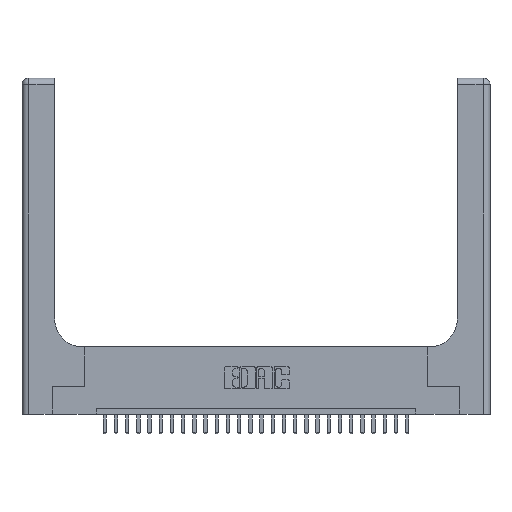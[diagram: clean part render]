
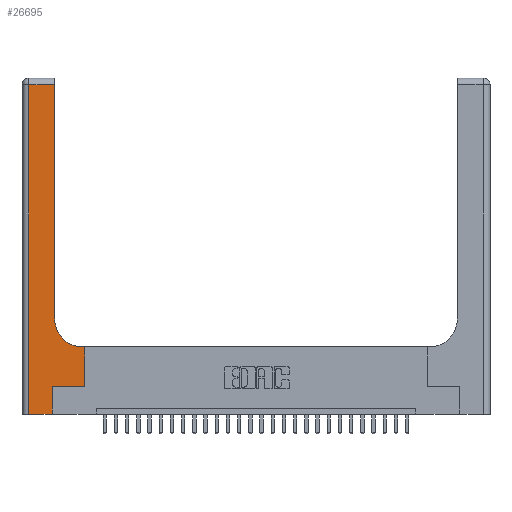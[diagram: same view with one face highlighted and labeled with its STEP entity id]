
A CAD part, top view. The second image highlights one B-rep face of the part: STEP entity #26695.
In plain terms, the highlighted planar face has unit normal (0, 0, 1).
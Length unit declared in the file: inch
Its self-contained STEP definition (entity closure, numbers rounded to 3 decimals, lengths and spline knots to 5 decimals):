
#1019 = ORIENTED_EDGE ( 'NONE', *, *, #23453, .T. ) ;
#1664 = ORIENTED_EDGE ( 'NONE', *, *, #26947, .T. ) ;
#1747 = DIRECTION ( 'NONE',  ( 1., 0., 0. ) ) ;
#2376 = LINE ( 'NONE', #21621, #3713 ) ;
#3713 = VECTOR ( 'NONE', #15261, 39.37008 ) ;
#3734 = CARTESIAN_POINT ( 'NONE',  ( 0.269, 0.25, 0.37 ) ) ;
#3906 = EDGE_CURVE ( 'NONE', #19540, #4794, #2376, .T. ) ;
#4467 = VECTOR ( 'NONE', #18921, 39.37008 ) ;
#4679 = VECTOR ( 'NONE', #12614, 39.37008 ) ;
#4794 = VERTEX_POINT ( 'NONE', #17191 ) ;
#4954 = EDGE_CURVE ( 'NONE', #4794, #5631, #6091, .T. ) ;
#5137 = ORIENTED_EDGE ( 'NONE', *, *, #26342, .T. ) ;
#5205 = DIRECTION ( 'NONE',  ( 0., 1., 0. ) ) ;
#5344 = CARTESIAN_POINT ( 'NONE',  ( 0.5415, 0.6, 0.37 ) ) ;
#5631 = VERTEX_POINT ( 'NONE', #7781 ) ;
#6091 = LINE ( 'NONE', #27931, #4679 ) ;
#6381 = DIRECTION ( 'NONE',  ( -1., 0., 0. ) ) ;
#7465 = VERTEX_POINT ( 'NONE', #10535 ) ;
#7767 = AXIS2_PLACEMENT_3D ( 'NONE', #19415, #8532, #6381 ) ;
#7781 = CARTESIAN_POINT ( 'NONE',  ( 0.269, 0., 0.37 ) ) ;
#8532 = DIRECTION ( 'NONE',  ( 0., 0., -1. ) ) ;
#9071 = DIRECTION ( 'NONE',  ( 0., 0., -1. ) ) ;
#9159 = DIRECTION ( 'NONE',  ( 1., 0., 0. ) ) ;
#9258 = EDGE_CURVE ( 'NONE', #5631, #19264, #20163, .T. ) ;
#9343 = LINE ( 'NONE', #24771, #26045 ) ;
#9934 = CARTESIAN_POINT ( 'NONE',  ( 0.06, 2.94, 0.37 ) ) ;
#10535 = CARTESIAN_POINT ( 'NONE',  ( 0.5585, 0.25, 0.37 ) ) ;
#10834 = CARTESIAN_POINT ( 'NONE',  ( 0.2915, 0.85, 0.37 ) ) ;
#10840 = DIRECTION ( 'NONE',  ( -1., 0., 0. ) ) ;
#11137 = ORIENTED_EDGE ( 'NONE', *, *, #9258, .T. ) ;
#11182 = ORIENTED_EDGE ( 'NONE', *, *, #4954, .T. ) ;
#12565 = LINE ( 'NONE', #18956, #19994 ) ;
#12614 = DIRECTION ( 'NONE',  ( 1., 0., 0. ) ) ;
#12843 = CARTESIAN_POINT ( 'NONE',  ( 0., 2.94, 0.37 ) ) ;
#13458 = VECTOR ( 'NONE', #5205, 39.37008 ) ;
#13619 = CARTESIAN_POINT ( 'NONE',  ( 0.5415, 0.85, 0.37 ) ) ;
#14384 = VERTEX_POINT ( 'NONE', #5344 ) ;
#14420 = VECTOR ( 'NONE', #10840, 39.37008 ) ;
#15104 = EDGE_CURVE ( 'NONE', #19264, #7465, #17779, .T. ) ;
#15176 = PLANE ( 'NONE',  #7767 ) ;
#15261 = DIRECTION ( 'NONE',  ( 0., -1., 0. ) ) ;
#16485 = CIRCLE ( 'NONE', #18891, 0.25 ) ;
#17094 = CARTESIAN_POINT ( 'NONE',  ( 0.5585, 0.6, 0.37 ) ) ;
#17191 = CARTESIAN_POINT ( 'NONE',  ( 0.06, 0., 0.37 ) ) ;
#17556 = CARTESIAN_POINT ( 'NONE',  ( 0.269, 0.25, 0.37 ) ) ;
#17679 = ORIENTED_EDGE ( 'NONE', *, *, #3906, .T. ) ;
#17779 = LINE ( 'NONE', #3734, #21870 ) ;
#18028 = VERTEX_POINT ( 'NONE', #10834 ) ;
#18075 = ORIENTED_EDGE ( 'NONE', *, *, #27725, .T. ) ;
#18619 = EDGE_LOOP ( 'NONE', ( #1019, #18075, #17679, #11182, #11137, #25982, #1664, #5137, #21457 ) ) ;
#18891 = AXIS2_PLACEMENT_3D ( 'NONE', #13619, #9071, #9159 ) ;
#18921 = DIRECTION ( 'NONE',  ( 0., 1., 0. ) ) ;
#18956 = CARTESIAN_POINT ( 'NONE',  ( 0.2915, 3., 0.37 ) ) ;
#19226 = LINE ( 'NONE', #20341, #13458 ) ;
#19264 = VERTEX_POINT ( 'NONE', #17556 ) ;
#19415 = CARTESIAN_POINT ( 'NONE',  ( 0., 3., 0.37 ) ) ;
#19540 = VERTEX_POINT ( 'NONE', #9934 ) ;
#19994 = VECTOR ( 'NONE', #27735, 39.37008 ) ;
#20163 = LINE ( 'NONE', #27996, #4467 ) ;
#20341 = CARTESIAN_POINT ( 'NONE',  ( 0.5585, 0.25, 0.37 ) ) ;
#20575 = VERTEX_POINT ( 'NONE', #25002 ) ;
#21457 = ORIENTED_EDGE ( 'NONE', *, *, #26749, .T. ) ;
#21553 = LINE ( 'NONE', #12843, #14420 ) ;
#21621 = CARTESIAN_POINT ( 'NONE',  ( 0.06, 3., 0.37 ) ) ;
#21870 = VECTOR ( 'NONE', #1747, 39.37008 ) ;
#23453 = EDGE_CURVE ( 'NONE', #18028, #20575, #12565, .T. ) ;
#23652 = FACE_OUTER_BOUND ( 'NONE', #18619, .T. ) ;
#24196 = VERTEX_POINT ( 'NONE', #17094 ) ;
#24771 = CARTESIAN_POINT ( 'NONE',  ( 0.2915, 0.6, 0.37 ) ) ;
#25002 = CARTESIAN_POINT ( 'NONE',  ( 0.2915, 2.94, 0.37 ) ) ;
#25982 = ORIENTED_EDGE ( 'NONE', *, *, #15104, .T. ) ;
#26045 = VECTOR ( 'NONE', #26954, 39.37008 ) ;
#26342 = EDGE_CURVE ( 'NONE', #24196, #14384, #9343, .T. ) ;
#26695 = ADVANCED_FACE ( 'NONE', ( #23652 ), #15176, .F. ) ;
#26749 = EDGE_CURVE ( 'NONE', #14384, #18028, #16485, .T. ) ;
#26947 = EDGE_CURVE ( 'NONE', #7465, #24196, #19226, .T. ) ;
#26954 = DIRECTION ( 'NONE',  ( -1., 0., 0. ) ) ;
#27725 = EDGE_CURVE ( 'NONE', #20575, #19540, #21553, .T. ) ;
#27735 = DIRECTION ( 'NONE',  ( 0., 1., 0. ) ) ;
#27931 = CARTESIAN_POINT ( 'NONE',  ( 0., 0., 0.37 ) ) ;
#27996 = CARTESIAN_POINT ( 'NONE',  ( 0.269, 0., 0.37 ) ) ;
